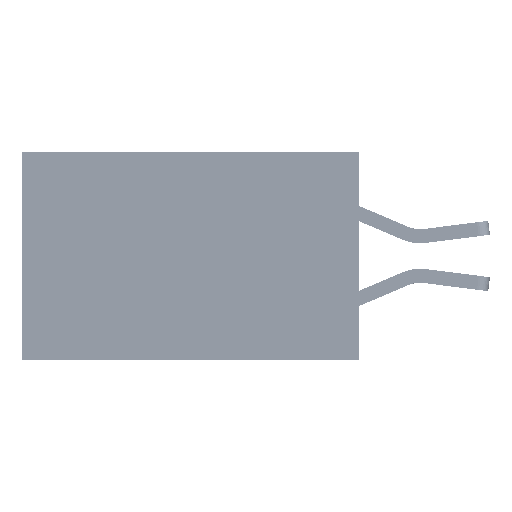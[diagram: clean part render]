
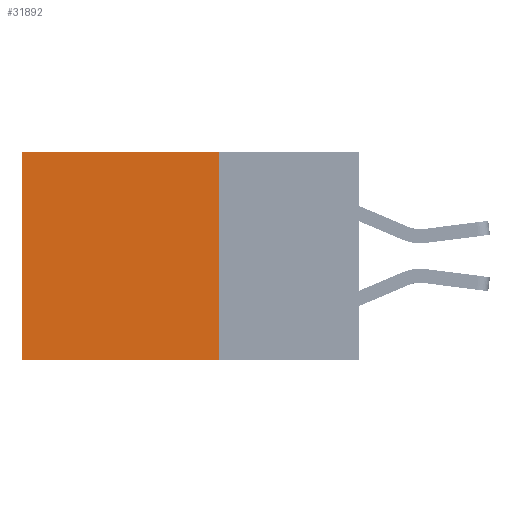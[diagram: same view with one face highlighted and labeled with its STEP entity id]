
A CAD part, left-side view. The second image highlights one B-rep face of the part: STEP entity #31892.
In plain terms, the highlighted planar face has unit normal (-1, 0, 0).
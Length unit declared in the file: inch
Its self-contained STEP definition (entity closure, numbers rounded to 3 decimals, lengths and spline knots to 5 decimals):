
#1518 = DIRECTION ( 'NONE',  ( 0., 0., -1. ) ) ;
#2242 = EDGE_CURVE ( 'NONE', #37330, #20558, #28146, .T. ) ;
#2708 = PLANE ( 'NONE',  #12450 ) ;
#3574 = VECTOR ( 'NONE', #1518, 39.37008 ) ;
#5328 = LINE ( 'NONE', #15239, #40424 ) ;
#7085 = ORIENTED_EDGE ( 'NONE', *, *, #24335, .F. ) ;
#7723 = VECTOR ( 'NONE', #45034, 39.37008 ) ;
#12242 = CARTESIAN_POINT ( 'NONE',  ( 0.2875, 0.25, -0.37 ) ) ;
#12450 = AXIS2_PLACEMENT_3D ( 'NONE', #45592, #23324, #33753 ) ;
#13957 = ORIENTED_EDGE ( 'NONE', *, *, #18295, .T. ) ;
#14036 = DIRECTION ( 'NONE',  ( 0., 0., -1. ) ) ;
#15239 = CARTESIAN_POINT ( 'NONE',  ( 0.2875, 0.25, -0.37 ) ) ;
#16206 = CARTESIAN_POINT ( 'NONE',  ( 0.2875, 0.25, 0. ) ) ;
#16417 = FACE_OUTER_BOUND ( 'NONE', #40713, .T. ) ;
#17001 = CARTESIAN_POINT ( 'NONE',  ( 0.2875, 0.25, 0. ) ) ;
#17618 = VERTEX_POINT ( 'NONE', #31053 ) ;
#18295 = EDGE_CURVE ( 'NONE', #17618, #37330, #39480, .T. ) ;
#18518 = DIRECTION ( 'NONE',  ( 0., 1., 0. ) ) ;
#20340 = EDGE_CURVE ( 'NONE', #17618, #28176, #43755, .T. ) ;
#20558 = VERTEX_POINT ( 'NONE', #43478 ) ;
#23324 = DIRECTION ( 'NONE',  ( 1., 0., 0. ) ) ;
#24335 = EDGE_CURVE ( 'NONE', #28176, #20558, #5328, .T. ) ;
#25411 = ORIENTED_EDGE ( 'NONE', *, *, #20340, .F. ) ;
#28146 = LINE ( 'NONE', #35653, #3574 ) ;
#28176 = VERTEX_POINT ( 'NONE', #12242 ) ;
#31053 = CARTESIAN_POINT ( 'NONE',  ( 0.2875, 0.25, 0. ) ) ;
#31892 = ADVANCED_FACE ( 'NONE', ( #16417 ), #2708, .F. ) ;
#33753 = DIRECTION ( 'NONE',  ( 0., 0., -1. ) ) ;
#35384 = VECTOR ( 'NONE', #14036, 39.37008 ) ;
#35653 = CARTESIAN_POINT ( 'NONE',  ( 0.2875, 0.6, 0. ) ) ;
#37330 = VERTEX_POINT ( 'NONE', #40619 ) ;
#39480 = LINE ( 'NONE', #16206, #7723 ) ;
#40065 = ORIENTED_EDGE ( 'NONE', *, *, #2242, .T. ) ;
#40424 = VECTOR ( 'NONE', #18518, 39.37008 ) ;
#40619 = CARTESIAN_POINT ( 'NONE',  ( 0.2875, 0.6, 0. ) ) ;
#40713 = EDGE_LOOP ( 'NONE', ( #40065, #7085, #25411, #13957 ) ) ;
#43478 = CARTESIAN_POINT ( 'NONE',  ( 0.2875, 0.6, -0.37 ) ) ;
#43755 = LINE ( 'NONE', #17001, #35384 ) ;
#45034 = DIRECTION ( 'NONE',  ( 0., 1., 0. ) ) ;
#45592 = CARTESIAN_POINT ( 'NONE',  ( 0.2875, 0.25, 0. ) ) ;
